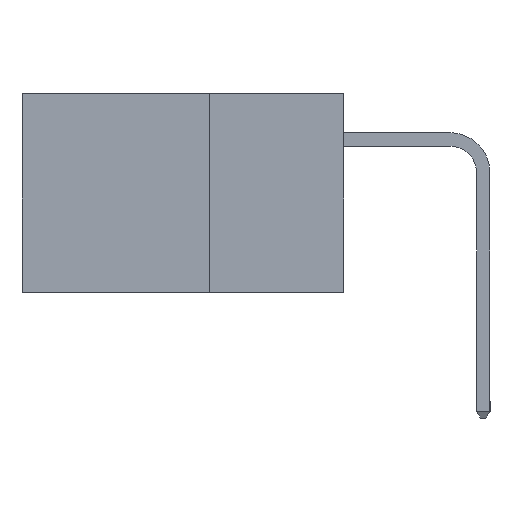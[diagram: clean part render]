
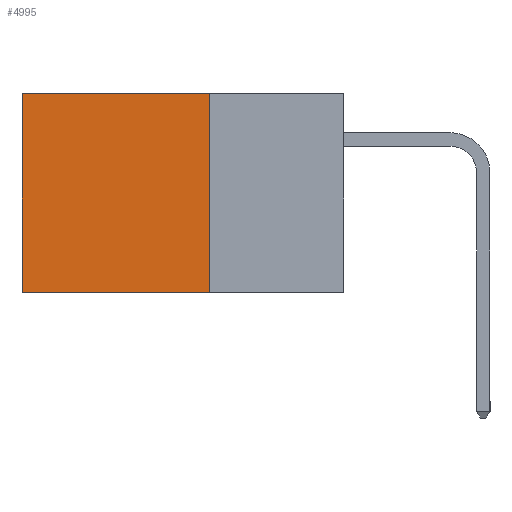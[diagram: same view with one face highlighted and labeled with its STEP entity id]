
A CAD part, left-side view. The second image highlights one B-rep face of the part: STEP entity #4995.
In plain terms, the highlighted planar face has unit normal (-1, 0, 0).
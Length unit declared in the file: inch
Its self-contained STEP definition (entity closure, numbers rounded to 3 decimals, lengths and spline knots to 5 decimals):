
#40 = LINE ( 'NONE', #8768, #13223 ) ;
#574 = VERTEX_POINT ( 'NONE', #9298 ) ;
#1080 = VECTOR ( 'NONE', #9661, 39.37008 ) ;
#1239 = CARTESIAN_POINT ( 'NONE',  ( 0.2615, 0.25, -0.37 ) ) ;
#1301 = EDGE_CURVE ( 'NONE', #574, #11550, #1855, .T. ) ;
#1451 = ORIENTED_EDGE ( 'NONE', *, *, #11137, .T. ) ;
#1855 = LINE ( 'NONE', #2507, #4430 ) ;
#2507 = CARTESIAN_POINT ( 'NONE',  ( 0.2615, 0.25, -0.37 ) ) ;
#2652 = CARTESIAN_POINT ( 'NONE',  ( 0.2615, 0.25, -0.37 ) ) ;
#2804 = ORIENTED_EDGE ( 'NONE', *, *, #6372, .T. ) ;
#4025 = LINE ( 'NONE', #1239, #1080 ) ;
#4364 = EDGE_LOOP ( 'NONE', ( #2804, #10270, #12421, #1451 ) ) ;
#4430 = VECTOR ( 'NONE', #7721, 39.37008 ) ;
#4995 = ADVANCED_FACE ( 'NONE', ( #5695 ), #11080, .F. ) ;
#5087 = DIRECTION ( 'NONE',  ( 1., 0., 0. ) ) ;
#5695 = FACE_OUTER_BOUND ( 'NONE', #4364, .T. ) ;
#5876 = VERTEX_POINT ( 'NONE', #10967 ) ;
#6255 = CARTESIAN_POINT ( 'NONE',  ( 0.2615, 0.25, 0. ) ) ;
#6276 = AXIS2_PLACEMENT_3D ( 'NONE', #9140, #5087, #12101 ) ;
#6372 = EDGE_CURVE ( 'NONE', #11628, #5876, #40, .T. ) ;
#6436 = LINE ( 'NONE', #6255, #11344 ) ;
#7289 = DIRECTION ( 'NONE',  ( 0., 1., 0. ) ) ;
#7721 = DIRECTION ( 'NONE',  ( 0., 0., -1. ) ) ;
#8768 = CARTESIAN_POINT ( 'NONE',  ( 0.2615, 0.6, -0.37 ) ) ;
#9140 = CARTESIAN_POINT ( 'NONE',  ( 0.2615, 0.25, -0.37 ) ) ;
#9298 = CARTESIAN_POINT ( 'NONE',  ( 0.2615, 0.25, 0. ) ) ;
#9661 = DIRECTION ( 'NONE',  ( 0., 1., 0. ) ) ;
#10270 = ORIENTED_EDGE ( 'NONE', *, *, #11920, .F. ) ;
#10967 = CARTESIAN_POINT ( 'NONE',  ( 0.2615, 0.6, -0.37 ) ) ;
#11080 = PLANE ( 'NONE',  #6276 ) ;
#11137 = EDGE_CURVE ( 'NONE', #574, #11628, #6436, .T. ) ;
#11344 = VECTOR ( 'NONE', #7289, 39.37008 ) ;
#11550 = VERTEX_POINT ( 'NONE', #2652 ) ;
#11628 = VERTEX_POINT ( 'NONE', #12952 ) ;
#11920 = EDGE_CURVE ( 'NONE', #11550, #5876, #4025, .T. ) ;
#12101 = DIRECTION ( 'NONE',  ( 0., 0., -1. ) ) ;
#12421 = ORIENTED_EDGE ( 'NONE', *, *, #1301, .F. ) ;
#12709 = DIRECTION ( 'NONE',  ( 0., 0., -1. ) ) ;
#12952 = CARTESIAN_POINT ( 'NONE',  ( 0.2615, 0.6, 0. ) ) ;
#13223 = VECTOR ( 'NONE', #12709, 39.37008 ) ;
